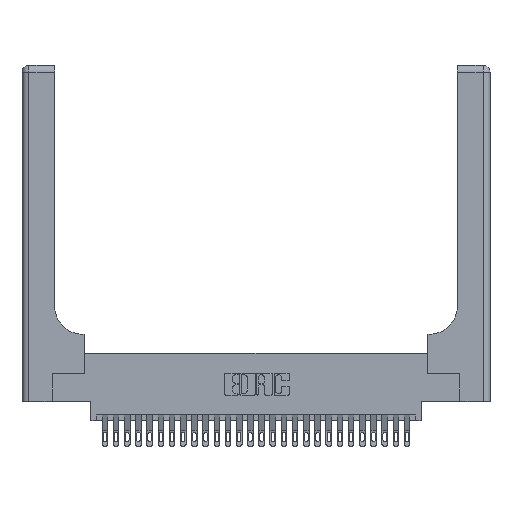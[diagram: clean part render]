
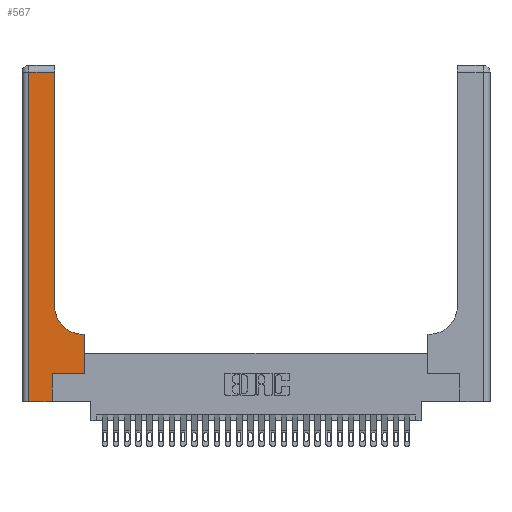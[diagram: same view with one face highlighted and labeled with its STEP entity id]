
A CAD part, top view. The second image highlights one B-rep face of the part: STEP entity #567.
In plain terms, the highlighted planar face has unit normal (0, 0, 1).
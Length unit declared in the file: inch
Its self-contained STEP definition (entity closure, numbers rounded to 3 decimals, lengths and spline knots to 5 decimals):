
#11 = CARTESIAN_POINT ( 'NONE',  ( 0.2915, 0.85, 0.37 ) ) ;
#241 = LINE ( 'NONE', #14645, #19479 ) ;
#256 = VECTOR ( 'NONE', #5226, 39.37008 ) ;
#567 = ADVANCED_FACE ( 'NONE', ( #21511 ), #3046, .F. ) ;
#645 = EDGE_CURVE ( 'NONE', #16112, #14393, #26845, .T. ) ;
#796 = VERTEX_POINT ( 'NONE', #18091 ) ;
#1521 = CARTESIAN_POINT ( 'NONE',  ( 0.06, 0., 0.37 ) ) ;
#1638 = CARTESIAN_POINT ( 'NONE',  ( 0.5415, 0.6, 0.37 ) ) ;
#1642 = CARTESIAN_POINT ( 'NONE',  ( 0., 2.94, 0.37 ) ) ;
#2356 = ORIENTED_EDGE ( 'NONE', *, *, #2514, .T. ) ;
#2514 = EDGE_CURVE ( 'NONE', #4919, #21324, #26989, .T. ) ;
#3046 = PLANE ( 'NONE',  #25603 ) ;
#3216 = EDGE_CURVE ( 'NONE', #14393, #28220, #3750, .T. ) ;
#3546 = CARTESIAN_POINT ( 'NONE',  ( 0.06, 3., 0.37 ) ) ;
#3750 = CIRCLE ( 'NONE', #10302, 0.25 ) ;
#4919 = VERTEX_POINT ( 'NONE', #27371 ) ;
#5147 = DIRECTION ( 'NONE',  ( -1., 0., 0. ) ) ;
#5226 = DIRECTION ( 'NONE',  ( 1., 0., 0. ) ) ;
#5557 = ORIENTED_EDGE ( 'NONE', *, *, #3216, .T. ) ;
#6130 = DIRECTION ( 'NONE',  ( 0., 0., -1. ) ) ;
#6152 = ORIENTED_EDGE ( 'NONE', *, *, #29261, .T. ) ;
#8149 = EDGE_CURVE ( 'NONE', #17844, #10644, #10614, .T. ) ;
#9432 = ORIENTED_EDGE ( 'NONE', *, *, #13777, .T. ) ;
#9478 = VECTOR ( 'NONE', #19786, 39.37008 ) ;
#10078 = DIRECTION ( 'NONE',  ( 1., 0., 0. ) ) ;
#10302 = AXIS2_PLACEMENT_3D ( 'NONE', #17589, #6130, #14992 ) ;
#10398 = CARTESIAN_POINT ( 'NONE',  ( 0.5585, 0.25, 0.37 ) ) ;
#10457 = VECTOR ( 'NONE', #19598, 39.37008 ) ;
#10614 = LINE ( 'NONE', #23753, #12392 ) ;
#10644 = VERTEX_POINT ( 'NONE', #23509 ) ;
#10799 = VECTOR ( 'NONE', #12621, 39.37008 ) ;
#11123 = ORIENTED_EDGE ( 'NONE', *, *, #8149, .T. ) ;
#11851 = DIRECTION ( 'NONE',  ( 0., 1., 0. ) ) ;
#11927 = EDGE_CURVE ( 'NONE', #10644, #4919, #241, .T. ) ;
#12232 = LINE ( 'NONE', #3546, #10457 ) ;
#12368 = DIRECTION ( 'NONE',  ( 0., 1., 0. ) ) ;
#12392 = VECTOR ( 'NONE', #10078, 39.37008 ) ;
#12432 = CARTESIAN_POINT ( 'NONE',  ( 0.2915, 0.6, 0.37 ) ) ;
#12621 = DIRECTION ( 'NONE',  ( -1., 0., 0. ) ) ;
#13007 = EDGE_LOOP ( 'NONE', ( #15721, #6152, #9432, #11123, #21023, #2356, #20883, #25537, #5557 ) ) ;
#13777 = EDGE_CURVE ( 'NONE', #25581, #17844, #12232, .T. ) ;
#14393 = VERTEX_POINT ( 'NONE', #1638 ) ;
#14645 = CARTESIAN_POINT ( 'NONE',  ( 0.269, 0., 0.37 ) ) ;
#14992 = DIRECTION ( 'NONE',  ( 1., 0., 0. ) ) ;
#15721 = ORIENTED_EDGE ( 'NONE', *, *, #19920, .T. ) ;
#16112 = VERTEX_POINT ( 'NONE', #23212 ) ;
#16833 = EDGE_CURVE ( 'NONE', #21324, #16112, #24680, .T. ) ;
#17167 = VECTOR ( 'NONE', #28638, 39.37008 ) ;
#17589 = CARTESIAN_POINT ( 'NONE',  ( 0.5415, 0.85, 0.37 ) ) ;
#17844 = VERTEX_POINT ( 'NONE', #1521 ) ;
#18091 = CARTESIAN_POINT ( 'NONE',  ( 0.2915, 2.94, 0.37 ) ) ;
#18191 = CARTESIAN_POINT ( 'NONE',  ( 0.06, 2.94, 0.37 ) ) ;
#18898 = CARTESIAN_POINT ( 'NONE',  ( 0.269, 0.25, 0.37 ) ) ;
#19479 = VECTOR ( 'NONE', #12368, 39.37008 ) ;
#19598 = DIRECTION ( 'NONE',  ( 0., -1., 0. ) ) ;
#19786 = DIRECTION ( 'NONE',  ( -1., 0., 0. ) ) ;
#19920 = EDGE_CURVE ( 'NONE', #28220, #796, #27012, .T. ) ;
#20883 = ORIENTED_EDGE ( 'NONE', *, *, #16833, .T. ) ;
#21023 = ORIENTED_EDGE ( 'NONE', *, *, #11927, .T. ) ;
#21228 = CARTESIAN_POINT ( 'NONE',  ( 0., 3., 0.37 ) ) ;
#21324 = VERTEX_POINT ( 'NONE', #23632 ) ;
#21429 = DIRECTION ( 'NONE',  ( 0., 0., -1. ) ) ;
#21511 = FACE_OUTER_BOUND ( 'NONE', #13007, .T. ) ;
#21965 = LINE ( 'NONE', #1642, #9478 ) ;
#23212 = CARTESIAN_POINT ( 'NONE',  ( 0.5585, 0.6, 0.37 ) ) ;
#23509 = CARTESIAN_POINT ( 'NONE',  ( 0.269, 0., 0.37 ) ) ;
#23632 = CARTESIAN_POINT ( 'NONE',  ( 0.5585, 0.25, 0.37 ) ) ;
#23753 = CARTESIAN_POINT ( 'NONE',  ( 0., 0., 0.37 ) ) ;
#24680 = LINE ( 'NONE', #10398, #17167 ) ;
#25537 = ORIENTED_EDGE ( 'NONE', *, *, #645, .T. ) ;
#25581 = VERTEX_POINT ( 'NONE', #18191 ) ;
#25603 = AXIS2_PLACEMENT_3D ( 'NONE', #21228, #21429, #5147 ) ;
#26845 = LINE ( 'NONE', #12432, #10799 ) ;
#26989 = LINE ( 'NONE', #18898, #256 ) ;
#27012 = LINE ( 'NONE', #27904, #27718 ) ;
#27371 = CARTESIAN_POINT ( 'NONE',  ( 0.269, 0.25, 0.37 ) ) ;
#27718 = VECTOR ( 'NONE', #11851, 39.37008 ) ;
#27904 = CARTESIAN_POINT ( 'NONE',  ( 0.2915, 3., 0.37 ) ) ;
#28220 = VERTEX_POINT ( 'NONE', #11 ) ;
#28638 = DIRECTION ( 'NONE',  ( 0., 1., 0. ) ) ;
#29261 = EDGE_CURVE ( 'NONE', #796, #25581, #21965, .T. ) ;
